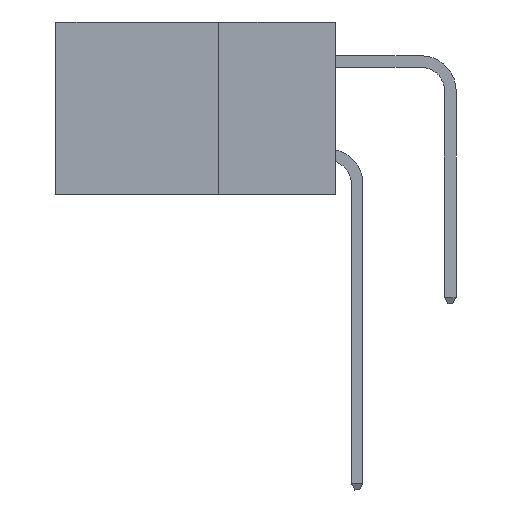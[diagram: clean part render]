
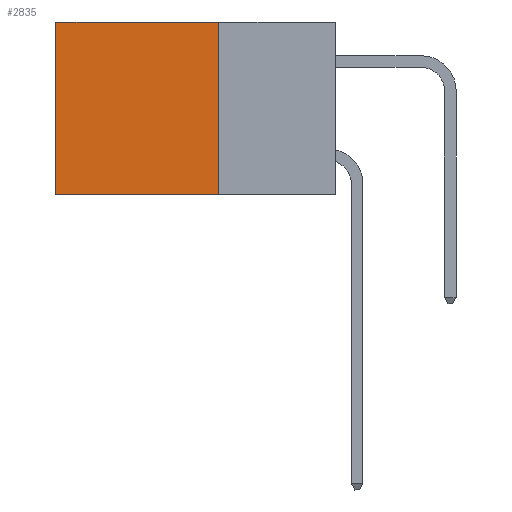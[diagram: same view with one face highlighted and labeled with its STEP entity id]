
A CAD part, left-side view. The second image highlights one B-rep face of the part: STEP entity #2835.
In plain terms, the highlighted planar face has unit normal (-1, 0, 0).
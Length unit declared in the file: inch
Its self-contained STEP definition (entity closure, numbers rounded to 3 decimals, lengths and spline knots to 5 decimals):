
#365 = ORIENTED_EDGE ( 'NONE', *, *, #15989, .F. ) ;
#727 = ORIENTED_EDGE ( 'NONE', *, *, #13958, .F. ) ;
#762 = LINE ( 'NONE', #13440, #16644 ) ;
#2456 = EDGE_LOOP ( 'NONE', ( #14882, #727, #365, #6855 ) ) ;
#2835 = ADVANCED_FACE ( 'NONE', ( #5656 ), #11246, .F. ) ;
#2938 = AXIS2_PLACEMENT_3D ( 'NONE', #16841, #10053, #4266 ) ;
#3247 = CARTESIAN_POINT ( 'NONE',  ( 0.2875, 0.6, 0. ) ) ;
#4088 = VERTEX_POINT ( 'NONE', #16846 ) ;
#4266 = DIRECTION ( 'NONE',  ( 0., 0., -1. ) ) ;
#4691 = CARTESIAN_POINT ( 'NONE',  ( 0.2875, 0.25, 0. ) ) ;
#5013 = DIRECTION ( 'NONE',  ( 0., 1., 0. ) ) ;
#5474 = EDGE_CURVE ( 'NONE', #13689, #4088, #8256, .T. ) ;
#5656 = FACE_OUTER_BOUND ( 'NONE', #2456, .T. ) ;
#6452 = LINE ( 'NONE', #3247, #16910 ) ;
#6853 = VERTEX_POINT ( 'NONE', #9905 ) ;
#6855 = ORIENTED_EDGE ( 'NONE', *, *, #5474, .T. ) ;
#8077 = CARTESIAN_POINT ( 'NONE',  ( 0.2875, 0.25, 0. ) ) ;
#8256 = LINE ( 'NONE', #8077, #16791 ) ;
#9703 = CARTESIAN_POINT ( 'NONE',  ( 0.2875, 0.25, 0. ) ) ;
#9905 = CARTESIAN_POINT ( 'NONE',  ( 0.2875, 0.25, -0.37 ) ) ;
#10053 = DIRECTION ( 'NONE',  ( 1., 0., 0. ) ) ;
#10384 = LINE ( 'NONE', #4691, #13724 ) ;
#11003 = DIRECTION ( 'NONE',  ( 0., 1., 0. ) ) ;
#11246 = PLANE ( 'NONE',  #2938 ) ;
#12474 = EDGE_CURVE ( 'NONE', #4088, #15712, #6452, .T. ) ;
#13440 = CARTESIAN_POINT ( 'NONE',  ( 0.2875, 0.25, -0.37 ) ) ;
#13689 = VERTEX_POINT ( 'NONE', #9703 ) ;
#13724 = VECTOR ( 'NONE', #16989, 39.37008 ) ;
#13958 = EDGE_CURVE ( 'NONE', #6853, #15712, #762, .T. ) ;
#14882 = ORIENTED_EDGE ( 'NONE', *, *, #12474, .T. ) ;
#15712 = VERTEX_POINT ( 'NONE', #17555 ) ;
#15737 = DIRECTION ( 'NONE',  ( 0., 0., -1. ) ) ;
#15989 = EDGE_CURVE ( 'NONE', #13689, #6853, #10384, .T. ) ;
#16644 = VECTOR ( 'NONE', #5013, 39.37008 ) ;
#16791 = VECTOR ( 'NONE', #11003, 39.37008 ) ;
#16841 = CARTESIAN_POINT ( 'NONE',  ( 0.2875, 0.25, 0. ) ) ;
#16846 = CARTESIAN_POINT ( 'NONE',  ( 0.2875, 0.6, 0. ) ) ;
#16910 = VECTOR ( 'NONE', #15737, 39.37008 ) ;
#16989 = DIRECTION ( 'NONE',  ( 0., 0., -1. ) ) ;
#17555 = CARTESIAN_POINT ( 'NONE',  ( 0.2875, 0.6, -0.37 ) ) ;
